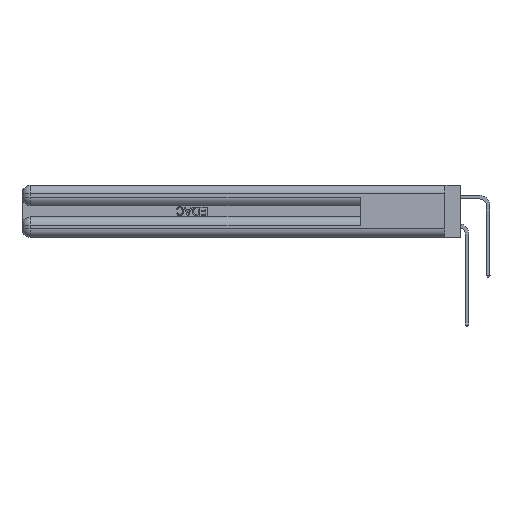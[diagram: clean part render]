
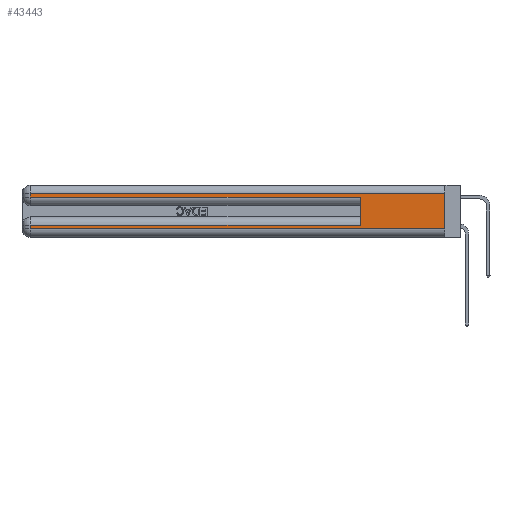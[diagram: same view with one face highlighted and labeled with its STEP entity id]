
A CAD part, left-side view. The second image highlights one B-rep face of the part: STEP entity #43443.
In plain terms, the highlighted planar face has unit normal (-1, 0, 0).
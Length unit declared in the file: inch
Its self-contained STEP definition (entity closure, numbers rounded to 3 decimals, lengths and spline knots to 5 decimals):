
#307 = CARTESIAN_POINT ( 'NONE',  ( 0., 0., 0.06 ) ) ;
#370 = VERTEX_POINT ( 'NONE', #307 ) ;
#673 = CARTESIAN_POINT ( 'NONE',  ( 0., 0.6, 0.085 ) ) ;
#1000 = DIRECTION ( 'NONE',  ( 0., 1., 0. ) ) ;
#1010 = CARTESIAN_POINT ( 'NONE',  ( 0., 2.94, 0.37 ) ) ;
#1528 = DIRECTION ( 'NONE',  ( 0., 0., -1. ) ) ;
#1846 = FACE_OUTER_BOUND ( 'NONE', #22332, .T. ) ;
#3721 = VERTEX_POINT ( 'NONE', #26721 ) ;
#3727 = LINE ( 'NONE', #19964, #6583 ) ;
#4878 = PLANE ( 'NONE',  #44120 ) ;
#5175 = EDGE_CURVE ( 'NONE', #3721, #23538, #19563, .T. ) ;
#5705 = EDGE_CURVE ( 'NONE', #38641, #3721, #32737, .T. ) ;
#6583 = VECTOR ( 'NONE', #1528, 39.37008 ) ;
#8564 = VECTOR ( 'NONE', #11810, 39.37008 ) ;
#9459 = DIRECTION ( 'NONE',  ( 0., -1., 0. ) ) ;
#10421 = DIRECTION ( 'NONE',  ( 0., 0., 1. ) ) ;
#11810 = DIRECTION ( 'NONE',  ( 0., 0., -1. ) ) ;
#13476 = EDGE_CURVE ( 'NONE', #47335, #35622, #41165, .T. ) ;
#14310 = CARTESIAN_POINT ( 'NONE',  ( 0., 0., 0.285 ) ) ;
#14431 = VECTOR ( 'NONE', #21600, 39.37008 ) ;
#16222 = DIRECTION ( 'NONE',  ( 0., 0., -1. ) ) ;
#16337 = EDGE_CURVE ( 'NONE', #35622, #30476, #29986, .T. ) ;
#18392 = ORIENTED_EDGE ( 'NONE', *, *, #19589, .F. ) ;
#19563 = LINE ( 'NONE', #27012, #8564 ) ;
#19589 = EDGE_CURVE ( 'NONE', #41970, #370, #3727, .T. ) ;
#19779 = CARTESIAN_POINT ( 'NONE',  ( 0., 0., 0.085 ) ) ;
#19964 = CARTESIAN_POINT ( 'NONE',  ( 0., 0., 0.37 ) ) ;
#21424 = LINE ( 'NONE', #37988, #24288 ) ;
#21600 = DIRECTION ( 'NONE',  ( 0., -1., 0. ) ) ;
#22177 = VECTOR ( 'NONE', #16222, 39.37008 ) ;
#22332 = EDGE_LOOP ( 'NONE', ( #18392, #31327, #34118, #32724, #38125, #32086, #25408, #31761 ) ) ;
#23538 = VERTEX_POINT ( 'NONE', #45328 ) ;
#24288 = VECTOR ( 'NONE', #41674, 39.37008 ) ;
#25408 = ORIENTED_EDGE ( 'NONE', *, *, #5175, .T. ) ;
#26721 = CARTESIAN_POINT ( 'NONE',  ( 0., 2.94, 0.085 ) ) ;
#27012 = CARTESIAN_POINT ( 'NONE',  ( 0., 2.94, 0.37 ) ) ;
#27322 = DIRECTION ( 'NONE',  ( 0., 0., -1. ) ) ;
#28436 = CARTESIAN_POINT ( 'NONE',  ( 0., 2.94, 0.285 ) ) ;
#29124 = EDGE_CURVE ( 'NONE', #23538, #370, #44666, .T. ) ;
#29163 = CARTESIAN_POINT ( 'NONE',  ( 0., 0.6, 0.145 ) ) ;
#29986 = LINE ( 'NONE', #14310, #14431 ) ;
#30476 = VERTEX_POINT ( 'NONE', #47046 ) ;
#31327 = ORIENTED_EDGE ( 'NONE', *, *, #44660, .T. ) ;
#31761 = ORIENTED_EDGE ( 'NONE', *, *, #29124, .T. ) ;
#31935 = CARTESIAN_POINT ( 'NONE',  ( 0., 0., 0.06 ) ) ;
#31997 = EDGE_CURVE ( 'NONE', #38641, #30476, #42733, .T. ) ;
#32086 = ORIENTED_EDGE ( 'NONE', *, *, #5705, .T. ) ;
#32724 = ORIENTED_EDGE ( 'NONE', *, *, #16337, .T. ) ;
#32737 = LINE ( 'NONE', #19779, #39686 ) ;
#33221 = VECTOR ( 'NONE', #9459, 39.37008 ) ;
#34118 = ORIENTED_EDGE ( 'NONE', *, *, #13476, .T. ) ;
#34647 = CARTESIAN_POINT ( 'NONE',  ( 0., 2.94, 0.31 ) ) ;
#35622 = VERTEX_POINT ( 'NONE', #28436 ) ;
#37988 = CARTESIAN_POINT ( 'NONE',  ( 0., 0., 0.31 ) ) ;
#38125 = ORIENTED_EDGE ( 'NONE', *, *, #31997, .F. ) ;
#38641 = VERTEX_POINT ( 'NONE', #673 ) ;
#39686 = VECTOR ( 'NONE', #1000, 39.37008 ) ;
#40034 = CARTESIAN_POINT ( 'NONE',  ( 0., 0., 0.31 ) ) ;
#41165 = LINE ( 'NONE', #1010, #22177 ) ;
#41674 = DIRECTION ( 'NONE',  ( 0., 1., 0. ) ) ;
#41970 = VERTEX_POINT ( 'NONE', #40034 ) ;
#42733 = LINE ( 'NONE', #29163, #46744 ) ;
#43443 = ADVANCED_FACE ( 'NONE', ( #1846 ), #4878, .F. ) ;
#44120 = AXIS2_PLACEMENT_3D ( 'NONE', #45445, #45599, #27322 ) ;
#44660 = EDGE_CURVE ( 'NONE', #41970, #47335, #21424, .T. ) ;
#44666 = LINE ( 'NONE', #31935, #33221 ) ;
#45328 = CARTESIAN_POINT ( 'NONE',  ( 0., 2.94, 0.06 ) ) ;
#45445 = CARTESIAN_POINT ( 'NONE',  ( 0., 0., 0.37 ) ) ;
#45599 = DIRECTION ( 'NONE',  ( 1., 0., 0. ) ) ;
#46744 = VECTOR ( 'NONE', #10421, 39.37008 ) ;
#47046 = CARTESIAN_POINT ( 'NONE',  ( 0., 0.6, 0.285 ) ) ;
#47335 = VERTEX_POINT ( 'NONE', #34647 ) ;
